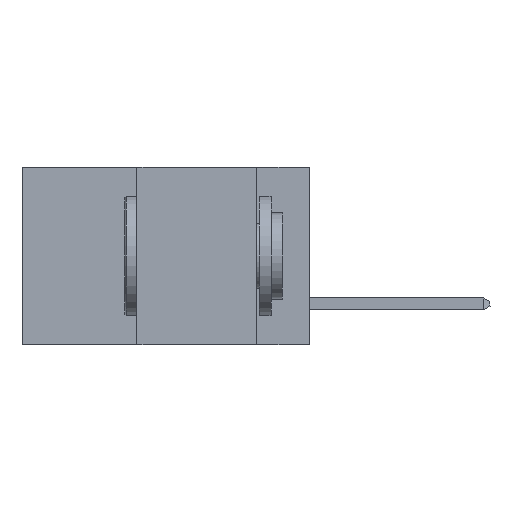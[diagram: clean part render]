
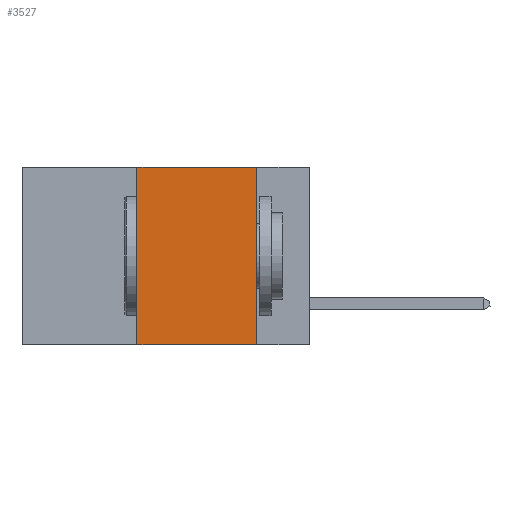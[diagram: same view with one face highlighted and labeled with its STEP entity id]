
A CAD part, left-side view. The second image highlights one B-rep face of the part: STEP entity #3527.
In plain terms, the highlighted planar face has unit normal (-1, 0, 0).
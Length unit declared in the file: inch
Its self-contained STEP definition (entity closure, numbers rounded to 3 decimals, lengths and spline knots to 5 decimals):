
#128 = CARTESIAN_POINT ( 'NONE',  ( 0., 0.36, -0.37 ) ) ;
#742 = EDGE_CURVE ( 'NONE', #26624, #27783, #2486, .T. ) ;
#1557 = FACE_OUTER_BOUND ( 'NONE', #18563, .T. ) ;
#2486 = LINE ( 'NONE', #9988, #20171 ) ;
#3306 = LINE ( 'NONE', #25503, #20998 ) ;
#3527 = ADVANCED_FACE ( 'NONE', ( #1557 ), #15384, .F. ) ;
#3595 = EDGE_CURVE ( 'NONE', #27783, #20775, #23897, .T. ) ;
#4060 = DIRECTION ( 'NONE',  ( 0., 0., -1. ) ) ;
#4530 = LINE ( 'NONE', #11560, #9957 ) ;
#6195 = CARTESIAN_POINT ( 'NONE',  ( 0., 0.6, 0. ) ) ;
#8877 = ORIENTED_EDGE ( 'NONE', *, *, #3595, .F. ) ;
#9394 = DIRECTION ( 'NONE',  ( 0., -1., 0. ) ) ;
#9957 = VECTOR ( 'NONE', #25359, 39.37008 ) ;
#9988 = CARTESIAN_POINT ( 'NONE',  ( 0., 0.6, 0. ) ) ;
#10097 = CARTESIAN_POINT ( 'NONE',  ( 0., 0.11, -0.37 ) ) ;
#10308 = DIRECTION ( 'NONE',  ( 0., -1., 0. ) ) ;
#10373 = EDGE_CURVE ( 'NONE', #14894, #20775, #3306, .T. ) ;
#10809 = DIRECTION ( 'NONE',  ( 1., 0., 0. ) ) ;
#11560 = CARTESIAN_POINT ( 'NONE',  ( 0., 0.36, 0. ) ) ;
#14220 = EDGE_CURVE ( 'NONE', #14894, #26624, #4530, .T. ) ;
#14894 = VERTEX_POINT ( 'NONE', #128 ) ;
#15384 = PLANE ( 'NONE',  #29014 ) ;
#18563 = EDGE_LOOP ( 'NONE', ( #8877, #25469, #25009, #21834 ) ) ;
#20171 = VECTOR ( 'NONE', #10308, 39.37008 ) ;
#20312 = CARTESIAN_POINT ( 'NONE',  ( 0., 0.11, 0. ) ) ;
#20775 = VERTEX_POINT ( 'NONE', #10097 ) ;
#20998 = VECTOR ( 'NONE', #9394, 39.37008 ) ;
#21834 = ORIENTED_EDGE ( 'NONE', *, *, #10373, .T. ) ;
#23897 = LINE ( 'NONE', #20312, #29361 ) ;
#25009 = ORIENTED_EDGE ( 'NONE', *, *, #14220, .F. ) ;
#25359 = DIRECTION ( 'NONE',  ( 0., 0., 1. ) ) ;
#25469 = ORIENTED_EDGE ( 'NONE', *, *, #742, .F. ) ;
#25503 = CARTESIAN_POINT ( 'NONE',  ( 0., 0.6, -0.37 ) ) ;
#26624 = VERTEX_POINT ( 'NONE', #28940 ) ;
#26968 = DIRECTION ( 'NONE',  ( 0., 0., -1. ) ) ;
#27783 = VERTEX_POINT ( 'NONE', #28927 ) ;
#28927 = CARTESIAN_POINT ( 'NONE',  ( 0., 0.11, 0. ) ) ;
#28940 = CARTESIAN_POINT ( 'NONE',  ( 0., 0.36, 0. ) ) ;
#29014 = AXIS2_PLACEMENT_3D ( 'NONE', #6195, #10809, #26968 ) ;
#29361 = VECTOR ( 'NONE', #4060, 39.37008 ) ;
